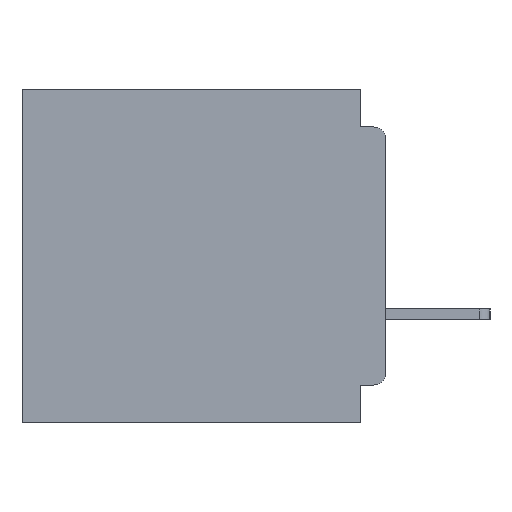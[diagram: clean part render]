
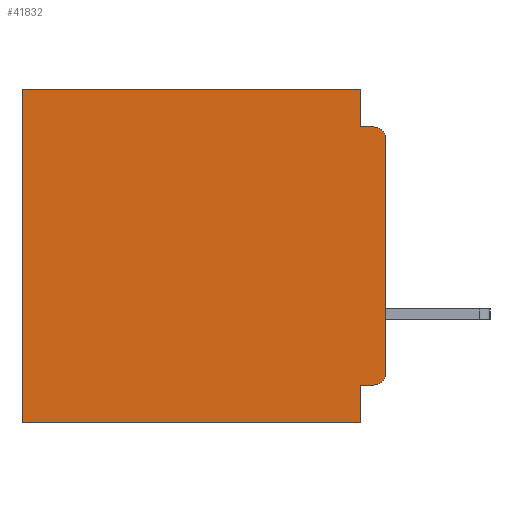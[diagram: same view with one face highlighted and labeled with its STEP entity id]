
A CAD part, left-side view. The second image highlights one B-rep face of the part: STEP entity #41832.
In plain terms, the highlighted planar face has unit normal (-1, 0, 0).
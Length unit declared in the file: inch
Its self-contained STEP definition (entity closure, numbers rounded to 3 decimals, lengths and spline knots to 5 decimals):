
#743 = VECTOR ( 'NONE', #41112, 39.37008 ) ;
#1070 = CARTESIAN_POINT ( 'NONE',  ( 0.3, 0.437, 0. ) ) ;
#1271 = CARTESIAN_POINT ( 'NONE',  ( 0.3, 0., -0.4 ) ) ;
#2053 = CARTESIAN_POINT ( 'NONE',  ( 0.3, 0., -0.4 ) ) ;
#2295 = DIRECTION ( 'NONE',  ( -1., 0., 0. ) ) ;
#2496 = CARTESIAN_POINT ( 'NONE',  ( 0.3, 0.031, -0.045 ) ) ;
#3065 = CARTESIAN_POINT ( 'NONE',  ( 0.3, 0.031, -0.4 ) ) ;
#3493 = ORIENTED_EDGE ( 'NONE', *, *, #54699, .T. ) ;
#3763 = EDGE_CURVE ( 'NONE', #12924, #54341, #39847, .T. ) ;
#4557 = ORIENTED_EDGE ( 'NONE', *, *, #26192, .T. ) ;
#5193 = LINE ( 'NONE', #17967, #56096 ) ;
#5350 = VERTEX_POINT ( 'NONE', #9884 ) ;
#6289 = DIRECTION ( 'NONE',  ( 0., 0., -1. ) ) ;
#6312 = CARTESIAN_POINT ( 'NONE',  ( 0.3, 0.031, -0.355 ) ) ;
#6550 = ORIENTED_EDGE ( 'NONE', *, *, #3763, .F. ) ;
#7871 = LINE ( 'NONE', #21680, #45610 ) ;
#8357 = VECTOR ( 'NONE', #36613, 39.37008 ) ;
#8942 = EDGE_CURVE ( 'NONE', #50068, #12924, #5193, .T. ) ;
#8975 = ORIENTED_EDGE ( 'NONE', *, *, #46169, .T. ) ;
#9884 = CARTESIAN_POINT ( 'NONE',  ( 0.3, 0.437, -0.4 ) ) ;
#10217 = VERTEX_POINT ( 'NONE', #61919 ) ;
#11066 = PLANE ( 'NONE',  #36067 ) ;
#12167 = VERTEX_POINT ( 'NONE', #43658 ) ;
#12924 = VERTEX_POINT ( 'NONE', #2496 ) ;
#13772 = DIRECTION ( 'NONE',  ( 0., 0., -1. ) ) ;
#14487 = ORIENTED_EDGE ( 'NONE', *, *, #39239, .F. ) ;
#15245 = VECTOR ( 'NONE', #63392, 39.37008 ) ;
#17281 = CARTESIAN_POINT ( 'NONE',  ( 0.3, 0., 0. ) ) ;
#17967 = CARTESIAN_POINT ( 'NONE',  ( 0.3, 0.031, 0. ) ) ;
#18691 = EDGE_LOOP ( 'NONE', ( #33292, #8975, #6550, #39957, #3493, #4557, #24237, #58117, #14487, #22580 ) ) ;
#19963 = LINE ( 'NONE', #2053, #8357 ) ;
#21109 = CARTESIAN_POINT ( 'NONE',  ( 0.3, 0.031, 0. ) ) ;
#21680 = CARTESIAN_POINT ( 'NONE',  ( 0.3, 0., -0.355 ) ) ;
#22580 = ORIENTED_EDGE ( 'NONE', *, *, #47232, .T. ) ;
#23637 = VECTOR ( 'NONE', #56673, 39.37008 ) ;
#24237 = ORIENTED_EDGE ( 'NONE', *, *, #36483, .F. ) ;
#24902 = EDGE_CURVE ( 'NONE', #46473, #31960, #45635, .T. ) ;
#25496 = CARTESIAN_POINT ( 'NONE',  ( 0.3, 0., -0.34 ) ) ;
#26192 = EDGE_CURVE ( 'NONE', #33306, #5350, #43155, .T. ) ;
#26695 = DIRECTION ( 'NONE',  ( 0., 1., 0. ) ) ;
#28250 = AXIS2_PLACEMENT_3D ( 'NONE', #31953, #2295, #36845 ) ;
#28909 = CARTESIAN_POINT ( 'NONE',  ( 0.3, 0.015, -0.06 ) ) ;
#30710 = FACE_OUTER_BOUND ( 'NONE', #18691, .T. ) ;
#31278 = CARTESIAN_POINT ( 'NONE',  ( 0.3, 0., -0.4 ) ) ;
#31953 = CARTESIAN_POINT ( 'NONE',  ( 0.3, 0.015, -0.34 ) ) ;
#31960 = VERTEX_POINT ( 'NONE', #37826 ) ;
#32879 = DIRECTION ( 'NONE',  ( 0., 0., -1. ) ) ;
#33292 = ORIENTED_EDGE ( 'NONE', *, *, #44071, .F. ) ;
#33306 = VERTEX_POINT ( 'NONE', #1070 ) ;
#33820 = DIRECTION ( 'NONE',  ( 0., 0., -1. ) ) ;
#34179 = CARTESIAN_POINT ( 'NONE',  ( 0.3, 0.015, -0.045 ) ) ;
#35867 = DIRECTION ( 'NONE',  ( 1., 0., 0. ) ) ;
#36067 = AXIS2_PLACEMENT_3D ( 'NONE', #1271, #35867, #6289 ) ;
#36483 = EDGE_CURVE ( 'NONE', #31960, #5350, #54817, .T. ) ;
#36613 = DIRECTION ( 'NONE',  ( 0., 0., -1. ) ) ;
#36845 = DIRECTION ( 'NONE',  ( 0., 0., -1. ) ) ;
#37613 = DIRECTION ( 'NONE',  ( 0., 0., -1. ) ) ;
#37826 = CARTESIAN_POINT ( 'NONE',  ( 0.3, 0.031, -0.4 ) ) ;
#39239 = EDGE_CURVE ( 'NONE', #12167, #46473, #7871, .T. ) ;
#39847 = LINE ( 'NONE', #62807, #15245 ) ;
#39957 = ORIENTED_EDGE ( 'NONE', *, *, #8942, .F. ) ;
#41112 = DIRECTION ( 'NONE',  ( 0., 1., 0. ) ) ;
#41604 = VECTOR ( 'NONE', #13772, 39.37008 ) ;
#41832 = ADVANCED_FACE ( 'NONE', ( #30710 ), #11066, .F. ) ;
#43155 = LINE ( 'NONE', #62724, #41604 ) ;
#43658 = CARTESIAN_POINT ( 'NONE',  ( 0.3, 0.015, -0.355 ) ) ;
#44071 = EDGE_CURVE ( 'NONE', #10217, #49983, #19963, .T. ) ;
#45610 = VECTOR ( 'NONE', #26695, 39.37008 ) ;
#45635 = LINE ( 'NONE', #3065, #58764 ) ;
#46169 = EDGE_CURVE ( 'NONE', #10217, #54341, #57393, .T. ) ;
#46227 = AXIS2_PLACEMENT_3D ( 'NONE', #28909, #63140, #33820 ) ;
#46473 = VERTEX_POINT ( 'NONE', #6312 ) ;
#47232 = EDGE_CURVE ( 'NONE', #12167, #49983, #61022, .T. ) ;
#49764 = LINE ( 'NONE', #17281, #23637 ) ;
#49983 = VERTEX_POINT ( 'NONE', #25496 ) ;
#50068 = VERTEX_POINT ( 'NONE', #21109 ) ;
#54341 = VERTEX_POINT ( 'NONE', #34179 ) ;
#54699 = EDGE_CURVE ( 'NONE', #50068, #33306, #49764, .T. ) ;
#54817 = LINE ( 'NONE', #31278, #743 ) ;
#56096 = VECTOR ( 'NONE', #32879, 39.37008 ) ;
#56673 = DIRECTION ( 'NONE',  ( 0., 1., 0. ) ) ;
#57393 = CIRCLE ( 'NONE', #46227, 0.015 ) ;
#58117 = ORIENTED_EDGE ( 'NONE', *, *, #24902, .F. ) ;
#58764 = VECTOR ( 'NONE', #37613, 39.37008 ) ;
#61022 = CIRCLE ( 'NONE', #28250, 0.015 ) ;
#61919 = CARTESIAN_POINT ( 'NONE',  ( 0.3, 0., -0.06 ) ) ;
#62724 = CARTESIAN_POINT ( 'NONE',  ( 0.3, 0.437, -0.4 ) ) ;
#62807 = CARTESIAN_POINT ( 'NONE',  ( 0.3, 0., -0.045 ) ) ;
#63140 = DIRECTION ( 'NONE',  ( -1., 0., 0. ) ) ;
#63392 = DIRECTION ( 'NONE',  ( 0., -1., 0. ) ) ;
